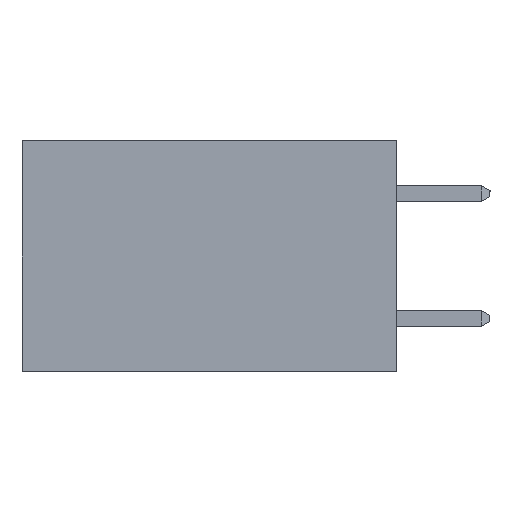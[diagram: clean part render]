
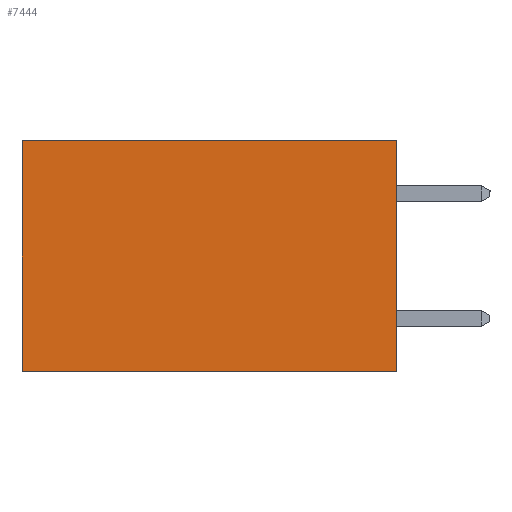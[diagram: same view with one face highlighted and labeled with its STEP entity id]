
A CAD part, left-side view. The second image highlights one B-rep face of the part: STEP entity #7444.
In plain terms, the highlighted planar face has unit normal (-1, 0, 0).
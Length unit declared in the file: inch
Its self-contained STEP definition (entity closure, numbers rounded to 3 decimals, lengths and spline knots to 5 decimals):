
#351 = EDGE_LOOP ( 'NONE', ( #22045, #12997, #5510, #9372 ) ) ;
#1261 = DIRECTION ( 'NONE',  ( 0., 1., 0. ) ) ;
#1289 = LINE ( 'NONE', #5311, #16253 ) ;
#1301 = DIRECTION ( 'NONE',  ( 0., 1., 0. ) ) ;
#3015 = LINE ( 'NONE', #20165, #22591 ) ;
#4200 = VERTEX_POINT ( 'NONE', #13242 ) ;
#4254 = EDGE_CURVE ( 'NONE', #13768, #9398, #15238, .T. ) ;
#5311 = CARTESIAN_POINT ( 'NONE',  ( 0.2615, 0.6, -0.37 ) ) ;
#5510 = ORIENTED_EDGE ( 'NONE', *, *, #4254, .F. ) ;
#6979 = CARTESIAN_POINT ( 'NONE',  ( 0.2615, 0., 0. ) ) ;
#7444 = ADVANCED_FACE ( 'NONE', ( #14806 ), #16914, .F. ) ;
#7457 = CARTESIAN_POINT ( 'NONE',  ( 0.2615, 0., 0. ) ) ;
#7841 = DIRECTION ( 'NONE',  ( 0., 0., -1. ) ) ;
#8732 = LINE ( 'NONE', #6979, #20662 ) ;
#9372 = ORIENTED_EDGE ( 'NONE', *, *, #12115, .T. ) ;
#9398 = VERTEX_POINT ( 'NONE', #21917 ) ;
#12115 = EDGE_CURVE ( 'NONE', #13768, #4200, #8732, .T. ) ;
#12997 = ORIENTED_EDGE ( 'NONE', *, *, #22181, .F. ) ;
#13242 = CARTESIAN_POINT ( 'NONE',  ( 0.2615, 0.6, 0. ) ) ;
#13697 = EDGE_CURVE ( 'NONE', #4200, #23410, #1289, .T. ) ;
#13768 = VERTEX_POINT ( 'NONE', #7457 ) ;
#14806 = FACE_OUTER_BOUND ( 'NONE', #351, .T. ) ;
#15176 = DIRECTION ( 'NONE',  ( 1., 0., 0. ) ) ;
#15238 = LINE ( 'NONE', #17237, #18684 ) ;
#16253 = VECTOR ( 'NONE', #16577, 39.37008 ) ;
#16577 = DIRECTION ( 'NONE',  ( 0., 0., -1. ) ) ;
#16914 = PLANE ( 'NONE',  #21506 ) ;
#17237 = CARTESIAN_POINT ( 'NONE',  ( 0.2615, 0., -0.37 ) ) ;
#18684 = VECTOR ( 'NONE', #7841, 39.37008 ) ;
#18909 = CARTESIAN_POINT ( 'NONE',  ( 0.2615, 0., -0.37 ) ) ;
#20165 = CARTESIAN_POINT ( 'NONE',  ( 0.2615, 0., -0.37 ) ) ;
#20662 = VECTOR ( 'NONE', #1301, 39.37008 ) ;
#21320 = CARTESIAN_POINT ( 'NONE',  ( 0.2615, 0.6, -0.37 ) ) ;
#21506 = AXIS2_PLACEMENT_3D ( 'NONE', #18909, #15176, #22809 ) ;
#21917 = CARTESIAN_POINT ( 'NONE',  ( 0.2615, 0., -0.37 ) ) ;
#22045 = ORIENTED_EDGE ( 'NONE', *, *, #13697, .T. ) ;
#22181 = EDGE_CURVE ( 'NONE', #9398, #23410, #3015, .T. ) ;
#22591 = VECTOR ( 'NONE', #1261, 39.37008 ) ;
#22809 = DIRECTION ( 'NONE',  ( 0., 0., -1. ) ) ;
#23410 = VERTEX_POINT ( 'NONE', #21320 ) ;
